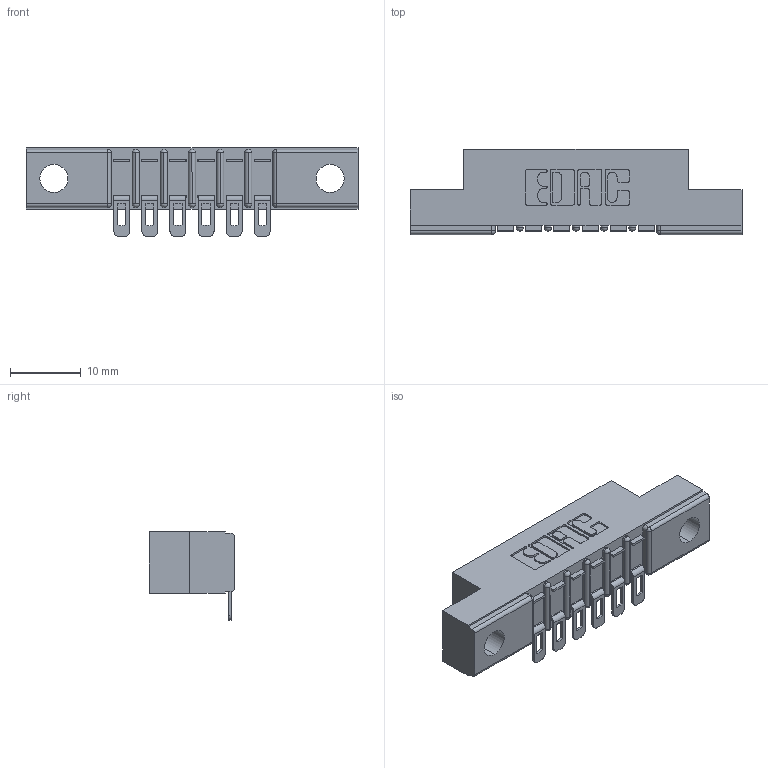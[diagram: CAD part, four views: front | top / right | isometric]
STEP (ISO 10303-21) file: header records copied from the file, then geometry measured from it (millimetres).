
FILE_DESCRIPTION (( 'STEP AP203' ), '1' );
FILE_NAME ('357-006-554-104.STEP', '2018-08-06T23:20:18', ( '' ), ( '' ), 'SwSTEP 2.0', 'SolidWorks 2016', '' );
FILE_SCHEMA (( 'CONFIG_CONTROL_DESIGN' ));
Length unit declared in the file: inch
Products named in the file (3): 307 Part_.156 Dia Mounting Holes; 307-290-002_554; 357-006-554-104
Assembly tree (7 placements, depth 2):
  357-006-554-104
    307 Part_.156 Dia Mounting Holes
    307-290-002_554  x6
Bounding box: 46.79 x 12.01 x 12.52 mm (x, y, z)
Volume: 2976.6 mm3; surface area: 4439.8 mm2
Topology: 7 solids, 7 shells, 625 faces, 1877 edges, 1230 vertices
Faces by surface type: plane 360, cylinder 251, sphere 14
Entity records: 10965 total; most frequent: CARTESIAN_POINT 1848, ORIENTED_EDGE 1836, DIRECTION 1810, EDGE_CURVE 918, LINE 686, VECTOR 686, VERTEX_POINT 600, AXIS2_PLACEMENT_3D 562
